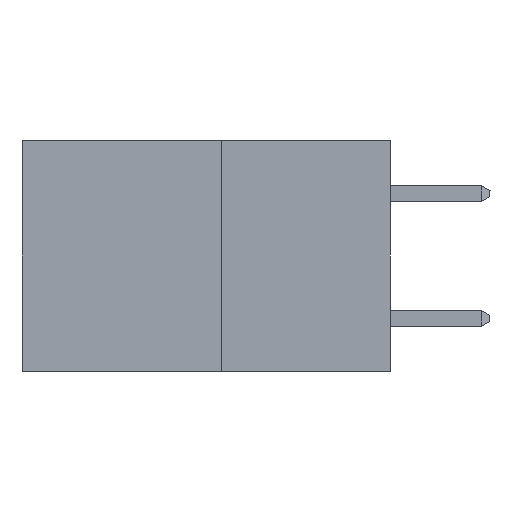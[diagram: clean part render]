
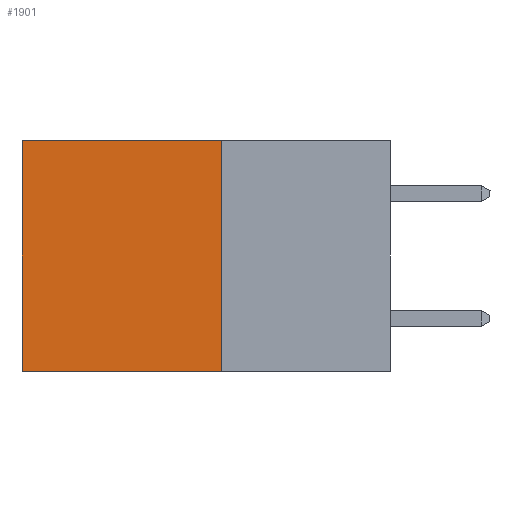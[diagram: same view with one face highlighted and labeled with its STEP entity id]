
A CAD part, left-side view. The second image highlights one B-rep face of the part: STEP entity #1901.
In plain terms, the highlighted planar face has unit normal (-1, 0, 0).
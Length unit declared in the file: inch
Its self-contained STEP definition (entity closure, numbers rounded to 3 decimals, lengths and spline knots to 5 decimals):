
#74 = DIRECTION ( 'NONE',  ( 1., 0., 0. ) ) ;
#345 = DIRECTION ( 'NONE',  ( 0., 0., -1. ) ) ;
#463 = LINE ( 'NONE', #652, #6211 ) ;
#652 = CARTESIAN_POINT ( 'NONE',  ( 0.277, 0.27, -0.37 ) ) ;
#903 = EDGE_CURVE ( 'NONE', #3246, #9565, #13931, .T. ) ;
#1901 = ADVANCED_FACE ( 'NONE', ( #14208 ), #7233, .F. ) ;
#3026 = CARTESIAN_POINT ( 'NONE',  ( 0.277, 0.27, 0. ) ) ;
#3102 = EDGE_LOOP ( 'NONE', ( #10017, #8925, #9410, #5727 ) ) ;
#3246 = VERTEX_POINT ( 'NONE', #14003 ) ;
#3325 = CARTESIAN_POINT ( 'NONE',  ( 0.277, 0.59, -0.37 ) ) ;
#3356 = DIRECTION ( 'NONE',  ( 0., 1., 0. ) ) ;
#4161 = CARTESIAN_POINT ( 'NONE',  ( 0.277, 0.27, 0. ) ) ;
#4213 = CARTESIAN_POINT ( 'NONE',  ( 0.277, 0.59, 0. ) ) ;
#5023 = VECTOR ( 'NONE', #3356, 39.37008 ) ;
#5727 = ORIENTED_EDGE ( 'NONE', *, *, #6375, .T. ) ;
#5741 = LINE ( 'NONE', #4161, #11486 ) ;
#5753 = LINE ( 'NONE', #9352, #8689 ) ;
#6211 = VECTOR ( 'NONE', #8572, 39.37008 ) ;
#6375 = EDGE_CURVE ( 'NONE', #9374, #9377, #5741, .T. ) ;
#7158 = AXIS2_PLACEMENT_3D ( 'NONE', #9839, #74, #8951 ) ;
#7233 = PLANE ( 'NONE',  #7158 ) ;
#8572 = DIRECTION ( 'NONE',  ( 0., 0., -1. ) ) ;
#8669 = EDGE_CURVE ( 'NONE', #9374, #3246, #463, .T. ) ;
#8689 = VECTOR ( 'NONE', #345, 39.37008 ) ;
#8925 = ORIENTED_EDGE ( 'NONE', *, *, #903, .F. ) ;
#8951 = DIRECTION ( 'NONE',  ( 0., 0., -1. ) ) ;
#9352 = CARTESIAN_POINT ( 'NONE',  ( 0.277, 0.59, -0.37 ) ) ;
#9374 = VERTEX_POINT ( 'NONE', #3026 ) ;
#9377 = VERTEX_POINT ( 'NONE', #4213 ) ;
#9410 = ORIENTED_EDGE ( 'NONE', *, *, #8669, .F. ) ;
#9565 = VERTEX_POINT ( 'NONE', #3325 ) ;
#9839 = CARTESIAN_POINT ( 'NONE',  ( 0.277, 0.27, -0.37 ) ) ;
#10017 = ORIENTED_EDGE ( 'NONE', *, *, #13361, .T. ) ;
#10552 = CARTESIAN_POINT ( 'NONE',  ( 0.277, 0.27, -0.37 ) ) ;
#10690 = DIRECTION ( 'NONE',  ( 0., 1., 0. ) ) ;
#11486 = VECTOR ( 'NONE', #10690, 39.37008 ) ;
#13361 = EDGE_CURVE ( 'NONE', #9377, #9565, #5753, .T. ) ;
#13931 = LINE ( 'NONE', #10552, #5023 ) ;
#14003 = CARTESIAN_POINT ( 'NONE',  ( 0.277, 0.27, -0.37 ) ) ;
#14208 = FACE_OUTER_BOUND ( 'NONE', #3102, .T. ) ;
